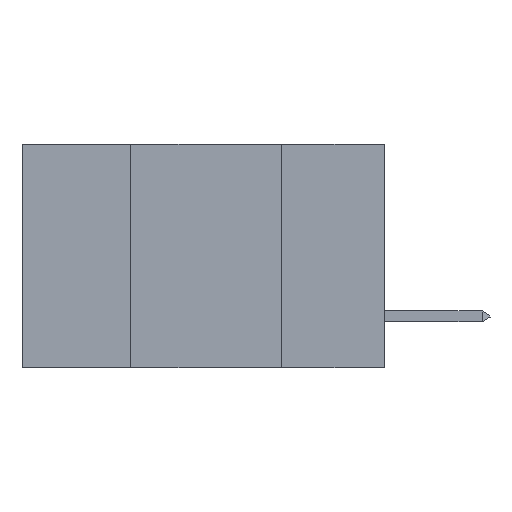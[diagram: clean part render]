
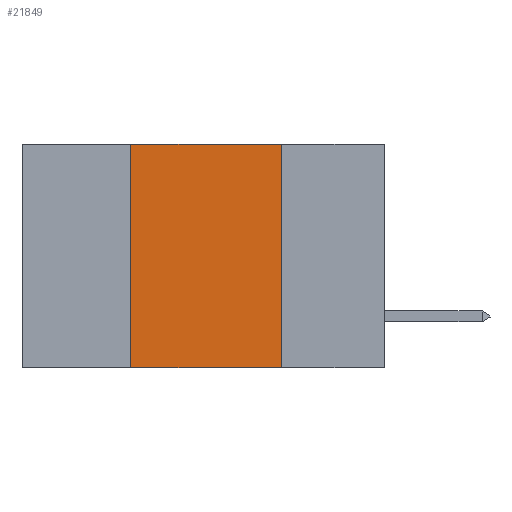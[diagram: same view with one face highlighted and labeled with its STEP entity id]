
A CAD part, left-side view. The second image highlights one B-rep face of the part: STEP entity #21849.
In plain terms, the highlighted planar face has unit normal (-1, 0, 0).
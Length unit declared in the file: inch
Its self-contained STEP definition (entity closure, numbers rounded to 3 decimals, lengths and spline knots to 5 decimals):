
#120 = VECTOR ( 'NONE', #4103, 39.37008 ) ;
#154 = LINE ( 'NONE', #3325, #26978 ) ;
#1300 = EDGE_CURVE ( 'NONE', #7403, #32545, #154, .T. ) ;
#1394 = CARTESIAN_POINT ( 'NONE',  ( 0., 0.42, 0. ) ) ;
#3325 = CARTESIAN_POINT ( 'NONE',  ( 0., 0.6, -0.37 ) ) ;
#4103 = DIRECTION ( 'NONE',  ( 0., 0., 1. ) ) ;
#4822 = DIRECTION ( 'NONE',  ( 0., -1., 0. ) ) ;
#5508 = CARTESIAN_POINT ( 'NONE',  ( 0., 0.17, -0.37 ) ) ;
#6947 = EDGE_LOOP ( 'NONE', ( #32119, #11038, #21405, #26647 ) ) ;
#7403 = VERTEX_POINT ( 'NONE', #22896 ) ;
#7887 = LINE ( 'NONE', #21124, #9956 ) ;
#8399 = DIRECTION ( 'NONE',  ( 0., -1., 0. ) ) ;
#9095 = VERTEX_POINT ( 'NONE', #23314 ) ;
#9956 = VECTOR ( 'NONE', #31623, 39.37008 ) ;
#11038 = ORIENTED_EDGE ( 'NONE', *, *, #18528, .F. ) ;
#18528 = EDGE_CURVE ( 'NONE', #21727, #9095, #25956, .T. ) ;
#21124 = CARTESIAN_POINT ( 'NONE',  ( 0., 0.17, 0. ) ) ;
#21403 = EDGE_CURVE ( 'NONE', #9095, #32545, #7887, .T. ) ;
#21405 = ORIENTED_EDGE ( 'NONE', *, *, #25176, .F. ) ;
#21727 = VERTEX_POINT ( 'NONE', #32818 ) ;
#21849 = ADVANCED_FACE ( 'NONE', ( #22698 ), #28187, .F. ) ;
#22698 = FACE_OUTER_BOUND ( 'NONE', #6947, .T. ) ;
#22848 = LINE ( 'NONE', #1394, #120 ) ;
#22861 = DIRECTION ( 'NONE',  ( 0., 0., -1. ) ) ;
#22896 = CARTESIAN_POINT ( 'NONE',  ( 0., 0.42, -0.37 ) ) ;
#23314 = CARTESIAN_POINT ( 'NONE',  ( 0., 0.17, 0. ) ) ;
#23950 = VECTOR ( 'NONE', #4822, 39.37008 ) ;
#25176 = EDGE_CURVE ( 'NONE', #7403, #21727, #22848, .T. ) ;
#25956 = LINE ( 'NONE', #27963, #23950 ) ;
#26647 = ORIENTED_EDGE ( 'NONE', *, *, #1300, .T. ) ;
#26978 = VECTOR ( 'NONE', #8399, 39.37008 ) ;
#27963 = CARTESIAN_POINT ( 'NONE',  ( 0., 0.6, 0. ) ) ;
#28187 = PLANE ( 'NONE',  #30908 ) ;
#30908 = AXIS2_PLACEMENT_3D ( 'NONE', #30936, #33366, #22861 ) ;
#30936 = CARTESIAN_POINT ( 'NONE',  ( 0., 0.6, 0. ) ) ;
#31623 = DIRECTION ( 'NONE',  ( 0., 0., -1. ) ) ;
#32119 = ORIENTED_EDGE ( 'NONE', *, *, #21403, .F. ) ;
#32545 = VERTEX_POINT ( 'NONE', #5508 ) ;
#32818 = CARTESIAN_POINT ( 'NONE',  ( 0., 0.42, 0. ) ) ;
#33366 = DIRECTION ( 'NONE',  ( 1., 0., 0. ) ) ;
